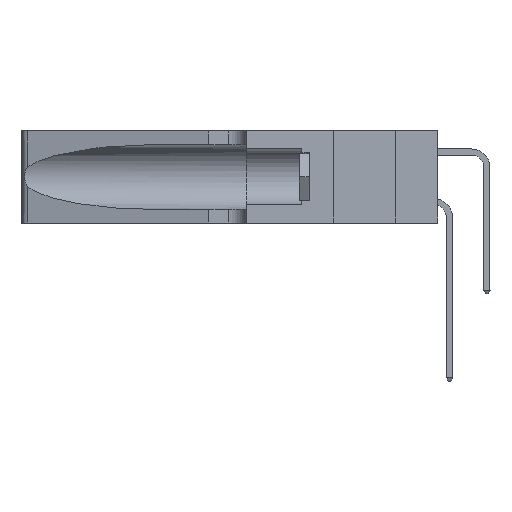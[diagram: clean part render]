
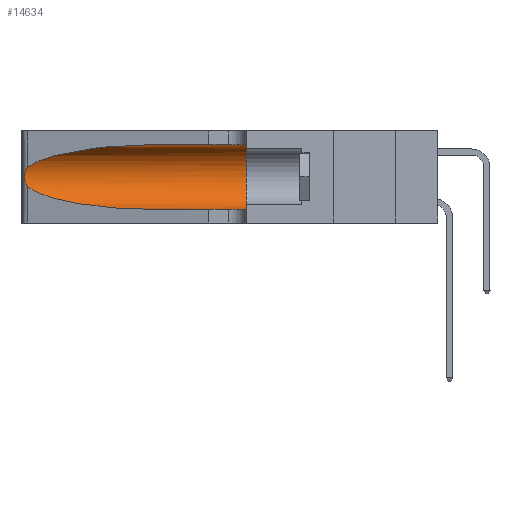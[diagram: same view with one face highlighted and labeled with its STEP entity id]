
A CAD part, left-side view. The second image highlights one B-rep face of the part: STEP entity #14634.
In plain terms, the highlighted cylindrical face has radius 3.308 mm (diameter 6.617 mm), a partial arc.
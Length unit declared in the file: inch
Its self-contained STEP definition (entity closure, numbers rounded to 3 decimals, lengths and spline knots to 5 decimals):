
#457 = AXIS2_PLACEMENT_3D ( 'NONE', #5922, #21198, #24070 ) ;
#573 = CARTESIAN_POINT ( 'NONE',  ( 0.1305, 0.72297, 0.31525 ) ) ;
#1045 = CARTESIAN_POINT ( 'NONE',  ( 0.25487, 1.22718, 0.14631 ) ) ;
#1403 = CARTESIAN_POINT ( 'NONE',  ( 0.1305, 0.72297, 0.05475 ) ) ;
#1770 = DIRECTION ( 'NONE',  ( 0., -1., 0. ) ) ;
#2225 = VERTEX_POINT ( 'NONE', #25121 ) ;
#2429 = CARTESIAN_POINT ( 'NONE',  ( 0.25787, 1.23484, 0.2124 ) ) ;
#3671 = CARTESIAN_POINT ( 'NONE',  ( 0.18966, 0.96281, 0.31525 ) ) ;
#5885 = VERTEX_POINT ( 'NONE', #7411 ) ;
#5922 = CARTESIAN_POINT ( 'NONE',  ( 0.1305, 1.61858, 0.185 ) ) ;
#6060 = CARTESIAN_POINT ( 'NONE',  ( 0.26018, 1.23835, 0.19895 ) ) ;
#6855 = CIRCLE ( 'NONE', #9257, 0.13025 ) ;
#6897 = VECTOR ( 'NONE', #1770, 39.37008 ) ;
#7375 = VERTEX_POINT ( 'NONE', #29792 ) ;
#7411 = CARTESIAN_POINT ( 'NONE',  ( 0.1305, 0.72297, 0.05475 ) ) ;
#7667 = CARTESIAN_POINT ( 'NONE',  ( 0.25555, 1.22994, 0.2215 ) ) ;
#8208 = ORIENTED_EDGE ( 'NONE', *, *, #22967, .T. ) ;
#8373 = ORIENTED_EDGE ( 'NONE', *, *, #31706, .F. ) ;
#8573 = CARTESIAN_POINT ( 'NONE',  ( 0.1305, 0.72297, 0.31525 ) ) ;
#8626 = CARTESIAN_POINT ( 'NONE',  ( 0.25856, 1.23593, 0.16098 ) ) ;
#8743 = CARTESIAN_POINT ( 'NONE',  ( 0.26075, 1.23896, 0.19203 ) ) ;
#9257 = AXIS2_PLACEMENT_3D ( 'NONE', #14079, #29865, #16680 ) ;
#9258 = CARTESIAN_POINT ( 'NONE',  ( 0.1305, 1.61858, 0.31525 ) ) ;
#9411 = EDGE_CURVE ( 'NONE', #7375, #15371, #21857, .T. ) ;
#10562 = EDGE_CURVE ( 'NONE', #15371, #5885, #24283, .T. ) ;
#10576 = CARTESIAN_POINT ( 'NONE',  ( 0.25487, 1.22718, 0.14631 ) ) ;
#11158 = CARTESIAN_POINT ( 'NONE',  ( 0.26017, 1.23833, 0.17102 ) ) ;
#12756 = VERTEX_POINT ( 'NONE', #21646 ) ;
#13310 = LINE ( 'NONE', #21102, #29776 ) ;
#14079 = CARTESIAN_POINT ( 'NONE',  ( 0.1305, 0.35, 0.185 ) ) ;
#14184 = CARTESIAN_POINT ( 'NONE',  ( 0.2373, 1.15595, 0.08982 ) ) ;
#14634 = ADVANCED_FACE ( 'NONE', ( #25140 ), #24308, .F. ) ;
#15371 = VERTEX_POINT ( 'NONE', #10576 ) ;
#16089 = CARTESIAN_POINT ( 'NONE',  ( 0.25789, 1.23486, 0.15765 ) ) ;
#16289 =( BOUNDED_CURVE ( )  B_SPLINE_CURVE ( 3, ( #8573, #3671, #16613, #21737 ),
 .UNSPECIFIED., .F., .T. ) 
 B_SPLINE_CURVE_WITH_KNOTS ( ( 4, 4 ),
 ( 1.5708, 2.84003 ),
 .UNSPECIFIED. ) 
 CURVE ( )  GEOMETRIC_REPRESENTATION_ITEM ( )  RATIONAL_B_SPLINE_CURVE ( ( 1., 0.87, 0.87, 1. ) ) 
 REPRESENTATION_ITEM ( '' )  );
#16613 = CARTESIAN_POINT ( 'NONE',  ( 0.2373, 1.15595, 0.28018 ) ) ;
#16678 = CARTESIAN_POINT ( 'NONE',  ( 0.25487, 1.22718, 0.14631 ) ) ;
#16680 = DIRECTION ( 'NONE',  ( 0., 0., 1. ) ) ;
#19934 = CARTESIAN_POINT ( 'NONE',  ( 0.25487, 1.22718, 0.22369 ) ) ;
#20678 = ORIENTED_EDGE ( 'NONE', *, *, #20932, .T. ) ;
#20778 = CARTESIAN_POINT ( 'NONE',  ( 0.25854, 1.2359, 0.20912 ) ) ;
#20813 = ORIENTED_EDGE ( 'NONE', *, *, #9411, .T. ) ;
#20932 = EDGE_CURVE ( 'NONE', #5885, #2225, #13310, .T. ) ;
#21102 = CARTESIAN_POINT ( 'NONE',  ( 0.1305, 1.61858, 0.05475 ) ) ;
#21198 = DIRECTION ( 'NONE',  ( 0., -1., 0. ) ) ;
#21210 = DIRECTION ( 'NONE',  ( 0., -1., 0. ) ) ;
#21572 = CARTESIAN_POINT ( 'NONE',  ( 0.18966, 0.96281, 0.05475 ) ) ;
#21646 = CARTESIAN_POINT ( 'NONE',  ( 0.1305, 0.35, 0.31525 ) ) ;
#21737 = CARTESIAN_POINT ( 'NONE',  ( 0.25487, 1.22718, 0.22369 ) ) ;
#21857 = B_SPLINE_CURVE_WITH_KNOTS ( 'NONE', 3,
 ( #19934, #7667, #30636, #2429, #20778, #6060, #8743, #28699, #11158, #8626, #16089, #29054, #31618, #1045 ),
 .UNSPECIFIED., .F., .F.,
 ( 4, 2, 2, 2, 2, 2, 4 ),
 ( 0., 0.00027, 0.00053, 0.00107, 0.0016, 0.00187, 0.00214 ),
 .UNSPECIFIED. ) ;
#22816 = ORIENTED_EDGE ( 'NONE', *, *, #10562, .T. ) ;
#22967 = EDGE_CURVE ( 'NONE', #25642, #7375, #16289, .T. ) ;
#23097 = EDGE_CURVE ( 'NONE', #25642, #12756, #32002, .T. ) ;
#24070 = DIRECTION ( 'NONE',  ( 0., 0., -1. ) ) ;
#24283 =( BOUNDED_CURVE ( )  B_SPLINE_CURVE ( 3, ( #16678, #14184, #21572, #1403 ),
 .UNSPECIFIED., .F., .T. ) 
 B_SPLINE_CURVE_WITH_KNOTS ( ( 4, 4 ),
 ( 3.44316, 4.71239 ),
 .UNSPECIFIED. ) 
 CURVE ( )  GEOMETRIC_REPRESENTATION_ITEM ( )  RATIONAL_B_SPLINE_CURVE ( ( 1., 0.87, 0.87, 1. ) ) 
 REPRESENTATION_ITEM ( '' )  );
#24308 = CYLINDRICAL_SURFACE ( 'NONE', #457, 0.13025 ) ;
#25121 = CARTESIAN_POINT ( 'NONE',  ( 0.1305, 0.35, 0.05475 ) ) ;
#25140 = FACE_OUTER_BOUND ( 'NONE', #30765, .T. ) ;
#25642 = VERTEX_POINT ( 'NONE', #573 ) ;
#27619 = ORIENTED_EDGE ( 'NONE', *, *, #23097, .F. ) ;
#28699 = CARTESIAN_POINT ( 'NONE',  ( 0.26075, 1.23896, 0.178 ) ) ;
#29054 = CARTESIAN_POINT ( 'NONE',  ( 0.25639, 1.23186, 0.15144 ) ) ;
#29776 = VECTOR ( 'NONE', #21210, 39.37008 ) ;
#29792 = CARTESIAN_POINT ( 'NONE',  ( 0.25487, 1.22718, 0.22369 ) ) ;
#29865 = DIRECTION ( 'NONE',  ( 0., 1., 0. ) ) ;
#30636 = CARTESIAN_POINT ( 'NONE',  ( 0.25639, 1.23184, 0.21858 ) ) ;
#30765 = EDGE_LOOP ( 'NONE', ( #8208, #20813, #22816, #20678, #8373, #27619 ) ) ;
#31618 = CARTESIAN_POINT ( 'NONE',  ( 0.25555, 1.22993, 0.14849 ) ) ;
#31706 = EDGE_CURVE ( 'NONE', #12756, #2225, #6855, .T. ) ;
#32002 = LINE ( 'NONE', #9258, #6897 ) ;
